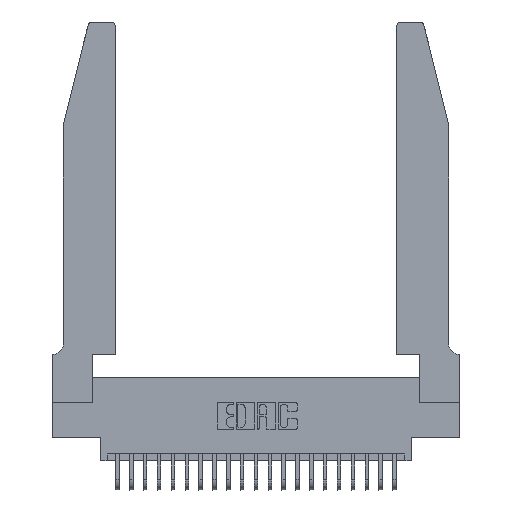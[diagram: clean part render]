
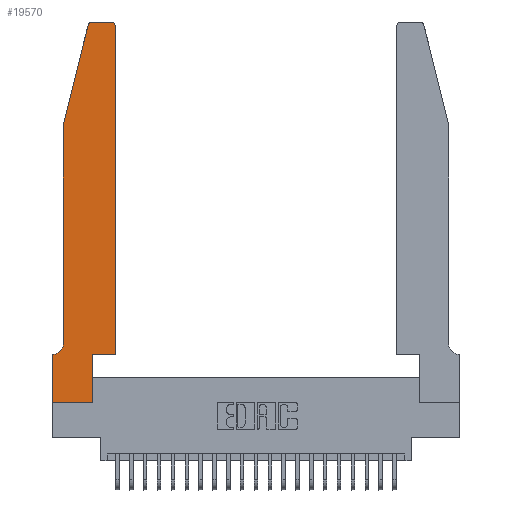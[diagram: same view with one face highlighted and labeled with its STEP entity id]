
A CAD part, top view. The second image highlights one B-rep face of the part: STEP entity #19570.
In plain terms, the highlighted planar face has unit normal (0, 0, 1).
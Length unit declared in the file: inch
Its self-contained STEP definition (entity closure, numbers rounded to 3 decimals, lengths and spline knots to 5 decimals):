
#543 = CARTESIAN_POINT ( 'NONE',  ( 0.0055, 0.42, 0.37 ) ) ;
#958 = PLANE ( 'NONE',  #6825 ) ;
#1050 = DIRECTION ( 'NONE',  ( 0., 0., 1. ) ) ;
#1154 = CARTESIAN_POINT ( 'NONE',  ( 0.2865, 0., 0.37 ) ) ;
#1165 = VERTEX_POINT ( 'NONE', #1154 ) ;
#1228 = VECTOR ( 'NONE', #12464, 39.37008 ) ;
#1329 = CARTESIAN_POINT ( 'NONE',  ( 0.0755, 0.35, 0.37 ) ) ;
#1530 = CARTESIAN_POINT ( 'NONE',  ( 0.0755, 2., 0.37 ) ) ;
#1553 = CARTESIAN_POINT ( 'NONE',  ( 0.0755, 2., 0.37 ) ) ;
#2010 = ORIENTED_EDGE ( 'NONE', *, *, #4880, .T. ) ;
#2467 = VECTOR ( 'NONE', #8723, 39.37008 ) ;
#2527 = CARTESIAN_POINT ( 'NONE',  ( 0.4505, 0.35, 0.37 ) ) ;
#2571 = DIRECTION ( 'NONE',  ( -1., 0., 0. ) ) ;
#2580 = VERTEX_POINT ( 'NONE', #21530 ) ;
#2688 = CARTESIAN_POINT ( 'NONE',  ( 0.2605, 2.75, 0.37 ) ) ;
#2700 = CARTESIAN_POINT ( 'NONE',  ( 0.2865, 0.35, 0.37 ) ) ;
#3594 = AXIS2_PLACEMENT_3D ( 'NONE', #8413, #22378, #10410 ) ;
#4094 = DIRECTION ( 'NONE',  ( 0., 1., 0. ) ) ;
#4096 = CARTESIAN_POINT ( 'NONE',  ( 0.4205, 2.75, 0.37 ) ) ;
#4260 = CARTESIAN_POINT ( 'NONE',  ( 0.2865, 0.35, 0.37 ) ) ;
#4595 = VECTOR ( 'NONE', #22523, 39.37008 ) ;
#4794 = LINE ( 'NONE', #2688, #25394 ) ;
#4880 = EDGE_CURVE ( 'NONE', #21090, #1165, #22494, .T. ) ;
#5609 = VERTEX_POINT ( 'NONE', #13211 ) ;
#5612 = CIRCLE ( 'NONE', #7433, 0.03 ) ;
#6163 = VECTOR ( 'NONE', #8962, 39.37008 ) ;
#6485 = LINE ( 'NONE', #9000, #16482 ) ;
#6715 = DIRECTION ( 'NONE',  ( -1., 0., 0. ) ) ;
#6781 = LINE ( 'NONE', #6953, #6163 ) ;
#6825 = AXIS2_PLACEMENT_3D ( 'NONE', #24965, #1050, #15007 ) ;
#6845 = ORIENTED_EDGE ( 'NONE', *, *, #25044, .T. ) ;
#6953 = CARTESIAN_POINT ( 'NONE',  ( 0., 0., 0.37 ) ) ;
#7168 = LINE ( 'NONE', #2700, #2467 ) ;
#7433 = AXIS2_PLACEMENT_3D ( 'NONE', #21741, #9749, #23717 ) ;
#7555 = ORIENTED_EDGE ( 'NONE', *, *, #12045, .T. ) ;
#7883 = EDGE_CURVE ( 'NONE', #23129, #11613, #4794, .T. ) ;
#8413 = CARTESIAN_POINT ( 'NONE',  ( 0.284, 2.72, 0.37 ) ) ;
#8723 = DIRECTION ( 'NONE',  ( 0., 1., 0. ) ) ;
#8962 = DIRECTION ( 'NONE',  ( 0., -1., 0. ) ) ;
#9000 = CARTESIAN_POINT ( 'NONE',  ( 0.0755, 2., 0.37 ) ) ;
#9081 = DIRECTION ( 'NONE',  ( -0.239, -0.971, 0. ) ) ;
#9367 = DIRECTION ( 'NONE',  ( -1., 0., 0. ) ) ;
#9749 = DIRECTION ( 'NONE',  ( 0., 0., 1. ) ) ;
#10410 = DIRECTION ( 'NONE',  ( 1., 0., 0. ) ) ;
#10602 = LINE ( 'NONE', #1553, #21248 ) ;
#11310 = VERTEX_POINT ( 'NONE', #19699 ) ;
#11613 = VERTEX_POINT ( 'NONE', #16522 ) ;
#12045 = EDGE_CURVE ( 'NONE', #11613, #2580, #17535, .T. ) ;
#12177 = ORIENTED_EDGE ( 'NONE', *, *, #20838, .T. ) ;
#12336 = EDGE_CURVE ( 'NONE', #14782, #17628, #10602, .T. ) ;
#12423 = VECTOR ( 'NONE', #9367, 39.37008 ) ;
#12426 = CARTESIAN_POINT ( 'NONE',  ( 0.4505, 2.72, 0.37 ) ) ;
#12455 = CARTESIAN_POINT ( 'NONE',  ( 0.0055, 0.35, 0.37 ) ) ;
#12464 = DIRECTION ( 'NONE',  ( 1., 0., 0. ) ) ;
#12732 = EDGE_CURVE ( 'NONE', #1165, #23703, #7168, .T. ) ;
#13046 = EDGE_CURVE ( 'NONE', #23768, #23129, #5612, .T. ) ;
#13081 = VECTOR ( 'NONE', #4094, 39.37008 ) ;
#13211 = CARTESIAN_POINT ( 'NONE',  ( 0.4505, 0.35, 0.37 ) ) ;
#13949 = LINE ( 'NONE', #2527, #4595 ) ;
#14173 = ORIENTED_EDGE ( 'NONE', *, *, #7883, .T. ) ;
#14513 = DIRECTION ( 'NONE',  ( 0., 0., -1. ) ) ;
#14529 = AXIS2_PLACEMENT_3D ( 'NONE', #543, #14513, #2571 ) ;
#14778 = ORIENTED_EDGE ( 'NONE', *, *, #13046, .T. ) ;
#14782 = VERTEX_POINT ( 'NONE', #1530 ) ;
#15007 = DIRECTION ( 'NONE',  ( 1., 0., 0. ) ) ;
#15202 = EDGE_CURVE ( 'NONE', #11310, #21090, #6781, .T. ) ;
#15541 = DIRECTION ( 'NONE',  ( 0., -1., 0. ) ) ;
#15725 = ORIENTED_EDGE ( 'NONE', *, *, #19039, .T. ) ;
#16482 = VECTOR ( 'NONE', #9081, 39.37008 ) ;
#16510 = ORIENTED_EDGE ( 'NONE', *, *, #12336, .T. ) ;
#16522 = CARTESIAN_POINT ( 'NONE',  ( 0.284, 2.75, 0.37 ) ) ;
#16879 = CARTESIAN_POINT ( 'NONE',  ( 0.0755, 0.42, 0.37 ) ) ;
#16914 = ORIENTED_EDGE ( 'NONE', *, *, #19575, .T. ) ;
#17535 = CIRCLE ( 'NONE', #3594, 0.03 ) ;
#17628 = VERTEX_POINT ( 'NONE', #16879 ) ;
#17733 = ORIENTED_EDGE ( 'NONE', *, *, #12732, .T. ) ;
#17794 = LINE ( 'NONE', #1329, #12423 ) ;
#17861 = EDGE_LOOP ( 'NONE', ( #14173, #7555, #16914, #16510, #22140, #15725, #20441, #2010, #17733, #12177, #6845, #14778 ) ) ;
#18462 = CARTESIAN_POINT ( 'NONE',  ( 0., 0., 0.37 ) ) ;
#18952 = CIRCLE ( 'NONE', #14529, 0.07 ) ;
#19039 = EDGE_CURVE ( 'NONE', #21308, #11310, #17794, .T. ) ;
#19077 = LINE ( 'NONE', #22024, #13081 ) ;
#19570 = ADVANCED_FACE ( 'NONE', ( #22407 ), #958, .T. ) ;
#19575 = EDGE_CURVE ( 'NONE', #2580, #14782, #6485, .T. ) ;
#19699 = CARTESIAN_POINT ( 'NONE',  ( 0., 0.35, 0.37 ) ) ;
#19860 = CARTESIAN_POINT ( 'NONE',  ( 0., 0., 0.37 ) ) ;
#20441 = ORIENTED_EDGE ( 'NONE', *, *, #15202, .T. ) ;
#20838 = EDGE_CURVE ( 'NONE', #23703, #5609, #13949, .T. ) ;
#21090 = VERTEX_POINT ( 'NONE', #19860 ) ;
#21248 = VECTOR ( 'NONE', #15541, 39.37008 ) ;
#21308 = VERTEX_POINT ( 'NONE', #12455 ) ;
#21530 = CARTESIAN_POINT ( 'NONE',  ( 0.25487, 2.72718, 0.37 ) ) ;
#21741 = CARTESIAN_POINT ( 'NONE',  ( 0.4205, 2.72, 0.37 ) ) ;
#21994 = EDGE_CURVE ( 'NONE', #17628, #21308, #18952, .T. ) ;
#22024 = CARTESIAN_POINT ( 'NONE',  ( 0.4505, 0.35, 0.37 ) ) ;
#22140 = ORIENTED_EDGE ( 'NONE', *, *, #21994, .T. ) ;
#22378 = DIRECTION ( 'NONE',  ( 0., 0., 1. ) ) ;
#22407 = FACE_OUTER_BOUND ( 'NONE', #17861, .T. ) ;
#22494 = LINE ( 'NONE', #18462, #1228 ) ;
#22523 = DIRECTION ( 'NONE',  ( 1., 0., 0. ) ) ;
#23129 = VERTEX_POINT ( 'NONE', #4096 ) ;
#23703 = VERTEX_POINT ( 'NONE', #4260 ) ;
#23717 = DIRECTION ( 'NONE',  ( 1., 0., 0. ) ) ;
#23768 = VERTEX_POINT ( 'NONE', #12426 ) ;
#24965 = CARTESIAN_POINT ( 'NONE',  ( 0., 0.35, 0.37 ) ) ;
#25044 = EDGE_CURVE ( 'NONE', #5609, #23768, #19077, .T. ) ;
#25394 = VECTOR ( 'NONE', #6715, 39.37008 ) ;
